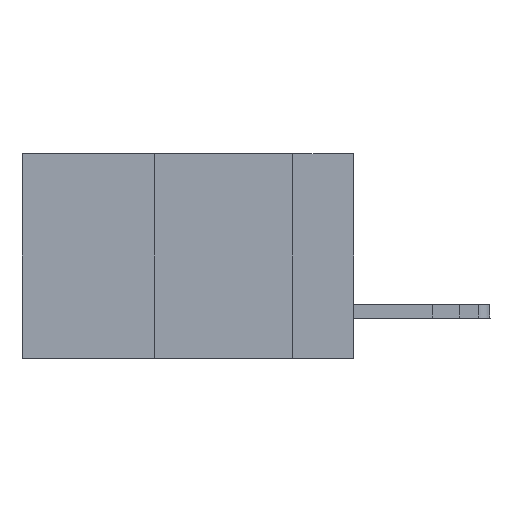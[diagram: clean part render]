
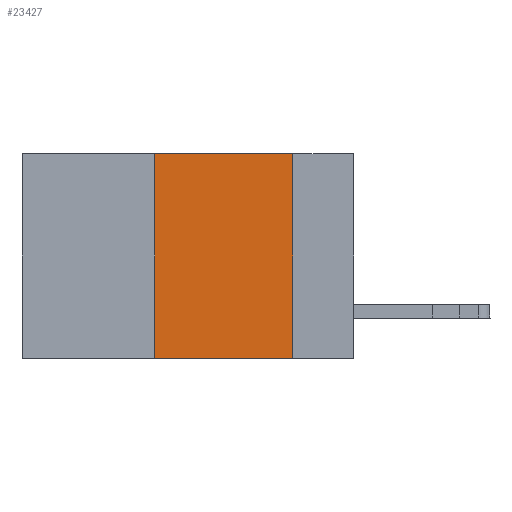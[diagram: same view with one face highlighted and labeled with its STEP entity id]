
A CAD part, left-side view. The second image highlights one B-rep face of the part: STEP entity #23427.
In plain terms, the highlighted planar face has unit normal (-1, 0, 0).
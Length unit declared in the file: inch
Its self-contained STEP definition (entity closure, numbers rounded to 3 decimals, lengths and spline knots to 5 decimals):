
#167 = VERTEX_POINT ( 'NONE', #4030 ) ;
#807 = EDGE_CURVE ( 'NONE', #6226, #167, #15783, .T. ) ;
#978 = LINE ( 'NONE', #8208, #22083 ) ;
#1829 = EDGE_CURVE ( 'NONE', #6900, #10893, #25452, .T. ) ;
#3759 = DIRECTION ( 'NONE',  ( 1., 0., 0. ) ) ;
#4030 = CARTESIAN_POINT ( 'NONE',  ( 0., 0.11, -0.37 ) ) ;
#6226 = VERTEX_POINT ( 'NONE', #24085 ) ;
#6415 = DIRECTION ( 'NONE',  ( 0., -1., 0. ) ) ;
#6494 = CARTESIAN_POINT ( 'NONE',  ( 0., 0.11, 0. ) ) ;
#6583 = EDGE_LOOP ( 'NONE', ( #10756, #12686, #8816, #22923 ) ) ;
#6900 = VERTEX_POINT ( 'NONE', #24438 ) ;
#7551 = CARTESIAN_POINT ( 'NONE',  ( 0., 0.6, 0. ) ) ;
#7641 = DIRECTION ( 'NONE',  ( 0., 0., -1. ) ) ;
#8208 = CARTESIAN_POINT ( 'NONE',  ( 0., 0.11, 0. ) ) ;
#8816 = ORIENTED_EDGE ( 'NONE', *, *, #22502, .F. ) ;
#9167 = VECTOR ( 'NONE', #22968, 39.37008 ) ;
#9567 = PLANE ( 'NONE',  #17349 ) ;
#10580 = VECTOR ( 'NONE', #15288, 39.37008 ) ;
#10756 = ORIENTED_EDGE ( 'NONE', *, *, #20197, .F. ) ;
#10893 = VERTEX_POINT ( 'NONE', #6494 ) ;
#12686 = ORIENTED_EDGE ( 'NONE', *, *, #1829, .F. ) ;
#14054 = FACE_OUTER_BOUND ( 'NONE', #6583, .T. ) ;
#15288 = DIRECTION ( 'NONE',  ( 0., -1., 0. ) ) ;
#15783 = LINE ( 'NONE', #20800, #25889 ) ;
#16145 = LINE ( 'NONE', #24864, #9167 ) ;
#17349 = AXIS2_PLACEMENT_3D ( 'NONE', #7551, #3759, #7641 ) ;
#19176 = CARTESIAN_POINT ( 'NONE',  ( 0., 0.6, 0. ) ) ;
#20197 = EDGE_CURVE ( 'NONE', #10893, #167, #978, .T. ) ;
#20800 = CARTESIAN_POINT ( 'NONE',  ( 0., 0.6, -0.37 ) ) ;
#22083 = VECTOR ( 'NONE', #24403, 39.37008 ) ;
#22502 = EDGE_CURVE ( 'NONE', #6226, #6900, #16145, .T. ) ;
#22923 = ORIENTED_EDGE ( 'NONE', *, *, #807, .T. ) ;
#22968 = DIRECTION ( 'NONE',  ( 0., 0., 1. ) ) ;
#23427 = ADVANCED_FACE ( 'NONE', ( #14054 ), #9567, .F. ) ;
#24085 = CARTESIAN_POINT ( 'NONE',  ( 0., 0.36, -0.37 ) ) ;
#24403 = DIRECTION ( 'NONE',  ( 0., 0., -1. ) ) ;
#24438 = CARTESIAN_POINT ( 'NONE',  ( 0., 0.36, 0. ) ) ;
#24864 = CARTESIAN_POINT ( 'NONE',  ( 0., 0.36, 0. ) ) ;
#25452 = LINE ( 'NONE', #19176, #10580 ) ;
#25889 = VECTOR ( 'NONE', #6415, 39.37008 ) ;
